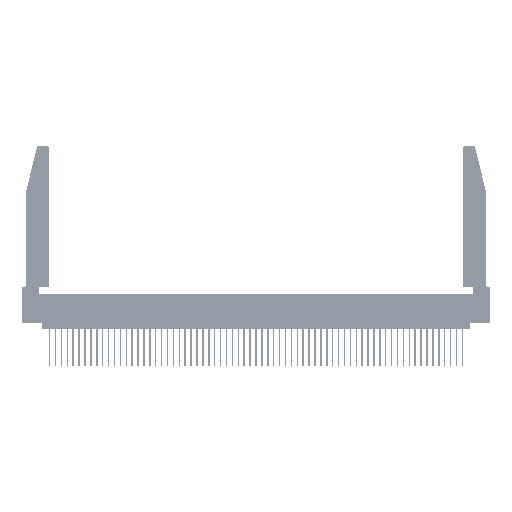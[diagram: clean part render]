
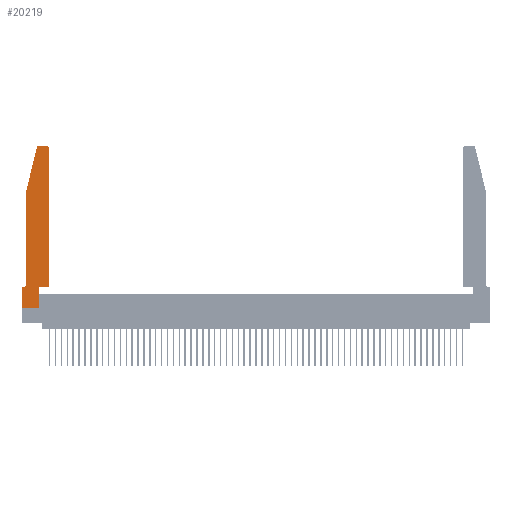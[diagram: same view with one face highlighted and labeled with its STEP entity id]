
A CAD part, top view. The second image highlights one B-rep face of the part: STEP entity #20219.
In plain terms, the highlighted planar face has unit normal (0, 0, 1).
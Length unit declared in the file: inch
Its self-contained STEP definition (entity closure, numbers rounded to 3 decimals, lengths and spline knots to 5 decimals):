
#640 = EDGE_CURVE ( 'NONE', #7147, #35938, #55174, .T. ) ;
#1287 = DIRECTION ( 'NONE',  ( 0., -1., 0. ) ) ;
#1377 = DIRECTION ( 'NONE',  ( 0., 0., -1. ) ) ;
#2284 = EDGE_CURVE ( 'NONE', #31683, #3254, #15369, .T. ) ;
#2318 = DIRECTION ( 'NONE',  ( -1., 0., 0. ) ) ;
#2812 = VECTOR ( 'NONE', #56082, 39.37008 ) ;
#3254 = VERTEX_POINT ( 'NONE', #56357 ) ;
#3904 = EDGE_CURVE ( 'NONE', #29334, #14806, #37774, .T. ) ;
#4600 = ORIENTED_EDGE ( 'NONE', *, *, #56220, .T. ) ;
#6088 = CARTESIAN_POINT ( 'NONE',  ( 0., 0., 0.37 ) ) ;
#7147 = VERTEX_POINT ( 'NONE', #47114 ) ;
#8883 = CARTESIAN_POINT ( 'NONE',  ( 0.2865, 0.35, 0.37 ) ) ;
#9440 = CARTESIAN_POINT ( 'NONE',  ( 0., 0., 0.37 ) ) ;
#9641 = DIRECTION ( 'NONE',  ( -1., 0., 0. ) ) ;
#10589 = CARTESIAN_POINT ( 'NONE',  ( 0.25487, 2.72718, 0.37 ) ) ;
#10661 = DIRECTION ( 'NONE',  ( 0., -1., 0. ) ) ;
#13676 = DIRECTION ( 'NONE',  ( 1., 0., 0. ) ) ;
#13679 = CARTESIAN_POINT ( 'NONE',  ( 0.0055, 0.35, 0.37 ) ) ;
#14078 = CARTESIAN_POINT ( 'NONE',  ( 0.2605, 2.75, 0.37 ) ) ;
#14806 = VERTEX_POINT ( 'NONE', #8883 ) ;
#15369 = LINE ( 'NONE', #27686, #16742 ) ;
#15918 = PLANE ( 'NONE',  #46602 ) ;
#16510 = ORIENTED_EDGE ( 'NONE', *, *, #41618, .T. ) ;
#16742 = VECTOR ( 'NONE', #1287, 39.37008 ) ;
#16755 = VECTOR ( 'NONE', #29477, 39.37008 ) ;
#17037 = ORIENTED_EDGE ( 'NONE', *, *, #3904, .T. ) ;
#17702 = CARTESIAN_POINT ( 'NONE',  ( 0.4505, 0.35, 0.37 ) ) ;
#20219 = ADVANCED_FACE ( 'NONE', ( #30846 ), #15918, .T. ) ;
#20344 = VECTOR ( 'NONE', #9641, 39.37008 ) ;
#20351 = LINE ( 'NONE', #35536, #42178 ) ;
#20368 = DIRECTION ( 'NONE',  ( 1., 0., 0. ) ) ;
#20893 = VECTOR ( 'NONE', #10661, 39.37008 ) ;
#21466 = CARTESIAN_POINT ( 'NONE',  ( 0.4505, 2.72, 0.37 ) ) ;
#21470 = VECTOR ( 'NONE', #48316, 39.37008 ) ;
#22017 = CIRCLE ( 'NONE', #41290, 0.07 ) ;
#23779 = ORIENTED_EDGE ( 'NONE', *, *, #30049, .T. ) ;
#24020 = DIRECTION ( 'NONE',  ( 0., 0., 1. ) ) ;
#24163 = DIRECTION ( 'NONE',  ( 0., 0., 1. ) ) ;
#25392 = AXIS2_PLACEMENT_3D ( 'NONE', #50129, #24020, #54510 ) ;
#25585 = EDGE_CURVE ( 'NONE', #37006, #51225, #56278, .T. ) ;
#26883 = VERTEX_POINT ( 'NONE', #10589 ) ;
#26979 = EDGE_CURVE ( 'NONE', #35581, #28529, #33753, .T. ) ;
#27121 = ORIENTED_EDGE ( 'NONE', *, *, #26979, .T. ) ;
#27686 = CARTESIAN_POINT ( 'NONE',  ( 0.0755, 2., 0.37 ) ) ;
#27783 = CARTESIAN_POINT ( 'NONE',  ( 0.0055, 0.42, 0.37 ) ) ;
#28529 = VERTEX_POINT ( 'NONE', #34038 ) ;
#28819 = LINE ( 'NONE', #47008, #50628 ) ;
#28902 = ORIENTED_EDGE ( 'NONE', *, *, #37132, .T. ) ;
#29334 = VERTEX_POINT ( 'NONE', #43958 ) ;
#29477 = DIRECTION ( 'NONE',  ( -0.239, -0.971, 0. ) ) ;
#30049 = EDGE_CURVE ( 'NONE', #14806, #37006, #20351, .T. ) ;
#30466 = ORIENTED_EDGE ( 'NONE', *, *, #25585, .T. ) ;
#30846 = FACE_OUTER_BOUND ( 'NONE', #46311, .T. ) ;
#31026 = VECTOR ( 'NONE', #2318, 39.37008 ) ;
#31522 = ORIENTED_EDGE ( 'NONE', *, *, #2284, .T. ) ;
#31683 = VERTEX_POINT ( 'NONE', #45460 ) ;
#31904 = EDGE_CURVE ( 'NONE', #26883, #31683, #40620, .T. ) ;
#32154 = DIRECTION ( 'NONE',  ( -1., 0., 0. ) ) ;
#33362 = ORIENTED_EDGE ( 'NONE', *, *, #640, .T. ) ;
#33491 = CIRCLE ( 'NONE', #43856, 0.03 ) ;
#33664 = CARTESIAN_POINT ( 'NONE',  ( 0.0755, 2., 0.37 ) ) ;
#33753 = LINE ( 'NONE', #37415, #31026 ) ;
#33900 = LINE ( 'NONE', #6088, #20893 ) ;
#34038 = CARTESIAN_POINT ( 'NONE',  ( 0., 0.35, 0.37 ) ) ;
#34659 = CIRCLE ( 'NONE', #25392, 0.03 ) ;
#35536 = CARTESIAN_POINT ( 'NONE',  ( 0.4505, 0.35, 0.37 ) ) ;
#35581 = VERTEX_POINT ( 'NONE', #13679 ) ;
#35938 = VERTEX_POINT ( 'NONE', #55137 ) ;
#36486 = ORIENTED_EDGE ( 'NONE', *, *, #40290, .T. ) ;
#37006 = VERTEX_POINT ( 'NONE', #44743 ) ;
#37132 = EDGE_CURVE ( 'NONE', #28529, #46595, #33900, .T. ) ;
#37415 = CARTESIAN_POINT ( 'NONE',  ( 0.0755, 0.35, 0.37 ) ) ;
#37774 = LINE ( 'NONE', #51720, #2812 ) ;
#38198 = DIRECTION ( 'NONE',  ( 1., 0., 0. ) ) ;
#38420 = ORIENTED_EDGE ( 'NONE', *, *, #53815, .T. ) ;
#40290 = EDGE_CURVE ( 'NONE', #3254, #35581, #22017, .T. ) ;
#40620 = LINE ( 'NONE', #33664, #16755 ) ;
#41290 = AXIS2_PLACEMENT_3D ( 'NONE', #27783, #1377, #32154 ) ;
#41618 = EDGE_CURVE ( 'NONE', #35938, #26883, #33491, .T. ) ;
#41928 = CARTESIAN_POINT ( 'NONE',  ( 0., 0.35, 0.37 ) ) ;
#42178 = VECTOR ( 'NONE', #13676, 39.37008 ) ;
#43856 = AXIS2_PLACEMENT_3D ( 'NONE', #50289, #24163, #54645 ) ;
#43958 = CARTESIAN_POINT ( 'NONE',  ( 0.2865, 0., 0.37 ) ) ;
#44743 = CARTESIAN_POINT ( 'NONE',  ( 0.4505, 0.35, 0.37 ) ) ;
#45460 = CARTESIAN_POINT ( 'NONE',  ( 0.0755, 2., 0.37 ) ) ;
#46311 = EDGE_LOOP ( 'NONE', ( #33362, #16510, #48437, #31522, #36486, #27121, #28902, #38420, #17037, #23779, #30466, #4600 ) ) ;
#46539 = DIRECTION ( 'NONE',  ( 0., 0., 1. ) ) ;
#46595 = VERTEX_POINT ( 'NONE', #9440 ) ;
#46602 = AXIS2_PLACEMENT_3D ( 'NONE', #41928, #46539, #20368 ) ;
#47008 = CARTESIAN_POINT ( 'NONE',  ( 0., 0., 0.37 ) ) ;
#47114 = CARTESIAN_POINT ( 'NONE',  ( 0.4205, 2.75, 0.37 ) ) ;
#48316 = DIRECTION ( 'NONE',  ( 0., 1., 0. ) ) ;
#48437 = ORIENTED_EDGE ( 'NONE', *, *, #31904, .T. ) ;
#50129 = CARTESIAN_POINT ( 'NONE',  ( 0.4205, 2.72, 0.37 ) ) ;
#50289 = CARTESIAN_POINT ( 'NONE',  ( 0.284, 2.72, 0.37 ) ) ;
#50628 = VECTOR ( 'NONE', #38198, 39.37008 ) ;
#51225 = VERTEX_POINT ( 'NONE', #21466 ) ;
#51720 = CARTESIAN_POINT ( 'NONE',  ( 0.2865, 0.35, 0.37 ) ) ;
#53815 = EDGE_CURVE ( 'NONE', #46595, #29334, #28819, .T. ) ;
#54510 = DIRECTION ( 'NONE',  ( 1., 0., 0. ) ) ;
#54645 = DIRECTION ( 'NONE',  ( 1., 0., 0. ) ) ;
#55137 = CARTESIAN_POINT ( 'NONE',  ( 0.284, 2.75, 0.37 ) ) ;
#55174 = LINE ( 'NONE', #14078, #20344 ) ;
#56082 = DIRECTION ( 'NONE',  ( 0., 1., 0. ) ) ;
#56220 = EDGE_CURVE ( 'NONE', #51225, #7147, #34659, .T. ) ;
#56278 = LINE ( 'NONE', #17702, #21470 ) ;
#56357 = CARTESIAN_POINT ( 'NONE',  ( 0.0755, 0.42, 0.37 ) ) ;
